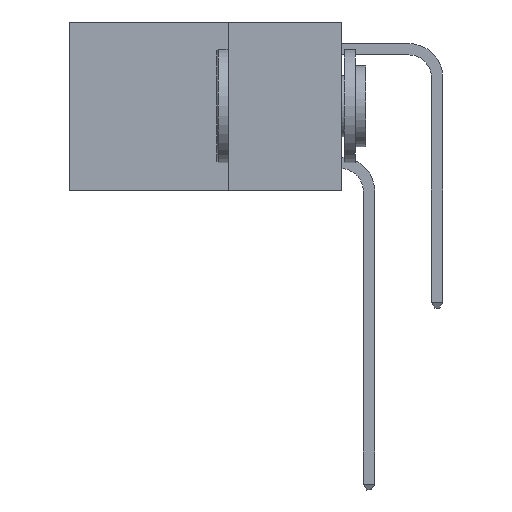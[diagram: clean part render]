
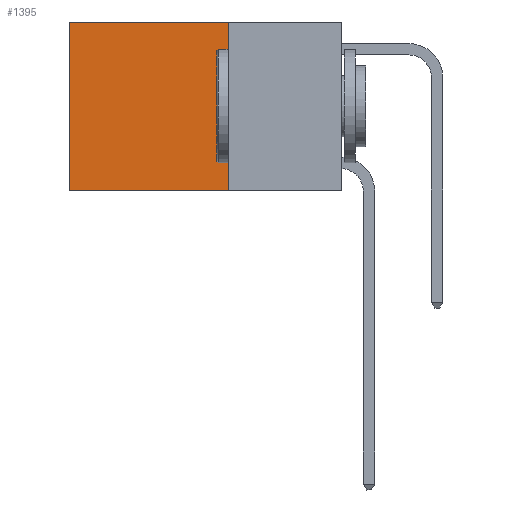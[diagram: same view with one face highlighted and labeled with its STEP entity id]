
A CAD part, left-side view. The second image highlights one B-rep face of the part: STEP entity #1395.
In plain terms, the highlighted planar face has unit normal (-1, 0, 0).
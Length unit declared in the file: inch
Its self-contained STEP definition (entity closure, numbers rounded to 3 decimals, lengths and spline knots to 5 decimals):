
#859 = CARTESIAN_POINT ( 'NONE',  ( 0.2625, 0.25, 0. ) ) ;
#1171 = LINE ( 'NONE', #2194, #10980 ) ;
#1395 = ADVANCED_FACE ( 'NONE', ( #11847 ), #10769, .F. ) ;
#1401 = ORIENTED_EDGE ( 'NONE', *, *, #3548, .T. ) ;
#1571 = DIRECTION ( 'NONE',  ( 0., 0., -1. ) ) ;
#1868 = CARTESIAN_POINT ( 'NONE',  ( 0.2625, 0.25, -0.37 ) ) ;
#1932 = CARTESIAN_POINT ( 'NONE',  ( 0.2625, 0.6, -0.37 ) ) ;
#2068 = EDGE_LOOP ( 'NONE', ( #4748, #14225, #4390, #1401 ) ) ;
#2194 = CARTESIAN_POINT ( 'NONE',  ( 0.2625, 0.25, 0. ) ) ;
#2679 = DIRECTION ( 'NONE',  ( 0., 1., 0. ) ) ;
#3006 = CARTESIAN_POINT ( 'NONE',  ( 0.2625, 0.6, 0. ) ) ;
#3548 = EDGE_CURVE ( 'NONE', #12460, #13504, #12557, .T. ) ;
#4078 = VERTEX_POINT ( 'NONE', #1932 ) ;
#4203 = VECTOR ( 'NONE', #2679, 39.37008 ) ;
#4228 = DIRECTION ( 'NONE',  ( 1., 0., 0. ) ) ;
#4390 = ORIENTED_EDGE ( 'NONE', *, *, #12724, .F. ) ;
#4438 = CARTESIAN_POINT ( 'NONE',  ( 0.2625, 0.25, 0. ) ) ;
#4645 = EDGE_CURVE ( 'NONE', #10659, #4078, #12779, .T. ) ;
#4683 = CARTESIAN_POINT ( 'NONE',  ( 0.2625, 0.25, 0. ) ) ;
#4748 = ORIENTED_EDGE ( 'NONE', *, *, #9836, .T. ) ;
#5639 = DIRECTION ( 'NONE',  ( 0., 0., -1. ) ) ;
#7209 = DIRECTION ( 'NONE',  ( 0., 1., 0. ) ) ;
#7323 = LINE ( 'NONE', #9351, #10349 ) ;
#7922 = CARTESIAN_POINT ( 'NONE',  ( 0.2625, 0.25, -0.37 ) ) ;
#9351 = CARTESIAN_POINT ( 'NONE',  ( 0.2625, 0.6, 0. ) ) ;
#9836 = EDGE_CURVE ( 'NONE', #13504, #4078, #7323, .T. ) ;
#10040 = VECTOR ( 'NONE', #7209, 39.37008 ) ;
#10349 = VECTOR ( 'NONE', #1571, 39.37008 ) ;
#10659 = VERTEX_POINT ( 'NONE', #7922 ) ;
#10769 = PLANE ( 'NONE',  #11388 ) ;
#10848 = DIRECTION ( 'NONE',  ( 0., 0., -1. ) ) ;
#10980 = VECTOR ( 'NONE', #5639, 39.37008 ) ;
#11388 = AXIS2_PLACEMENT_3D ( 'NONE', #859, #4228, #10848 ) ;
#11847 = FACE_OUTER_BOUND ( 'NONE', #2068, .T. ) ;
#12460 = VERTEX_POINT ( 'NONE', #4438 ) ;
#12557 = LINE ( 'NONE', #4683, #4203 ) ;
#12724 = EDGE_CURVE ( 'NONE', #12460, #10659, #1171, .T. ) ;
#12779 = LINE ( 'NONE', #1868, #10040 ) ;
#13504 = VERTEX_POINT ( 'NONE', #3006 ) ;
#14225 = ORIENTED_EDGE ( 'NONE', *, *, #4645, .F. ) ;
